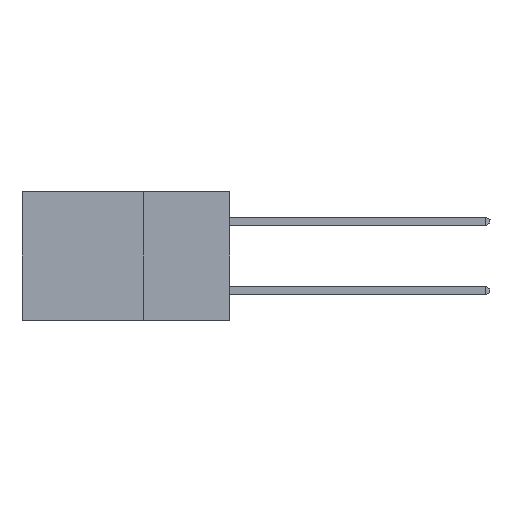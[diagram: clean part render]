
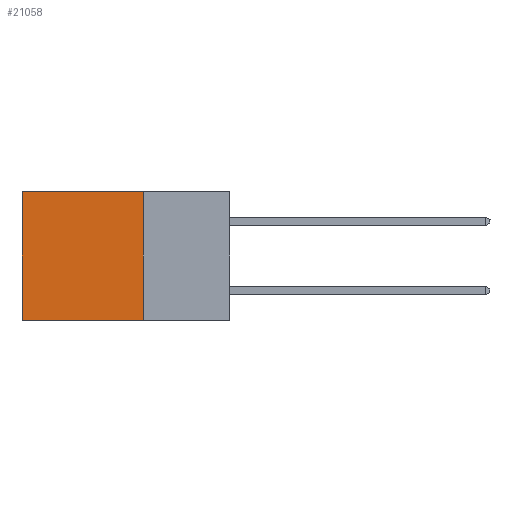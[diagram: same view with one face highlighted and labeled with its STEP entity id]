
A CAD part, left-side view. The second image highlights one B-rep face of the part: STEP entity #21058.
In plain terms, the highlighted planar face has unit normal (-1, 0, 0).
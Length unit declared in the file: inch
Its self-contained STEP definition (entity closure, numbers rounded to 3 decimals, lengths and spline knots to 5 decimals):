
#606 = DIRECTION ( 'NONE',  ( 0., 1., 0. ) ) ;
#782 = CARTESIAN_POINT ( 'NONE',  ( 0.298, 0.25, 0. ) ) ;
#2082 = VERTEX_POINT ( 'NONE', #9277 ) ;
#3116 = DIRECTION ( 'NONE',  ( 0., 0., -1. ) ) ;
#3853 = VECTOR ( 'NONE', #17124, 39.37008 ) ;
#4188 = ORIENTED_EDGE ( 'NONE', *, *, #10128, .F. ) ;
#5757 = VERTEX_POINT ( 'NONE', #782 ) ;
#6458 = CARTESIAN_POINT ( 'NONE',  ( 0.298, 0.6, 0. ) ) ;
#6996 = VERTEX_POINT ( 'NONE', #15014 ) ;
#7522 = LINE ( 'NONE', #8868, #10179 ) ;
#8371 = AXIS2_PLACEMENT_3D ( 'NONE', #20849, #12658, #12374 ) ;
#8868 = CARTESIAN_POINT ( 'NONE',  ( 0.298, 0.25, 0. ) ) ;
#9277 = CARTESIAN_POINT ( 'NONE',  ( 0.298, 0.6, -0.37 ) ) ;
#9330 = LINE ( 'NONE', #12622, #3853 ) ;
#9801 = DIRECTION ( 'NONE',  ( 0., 0., -1. ) ) ;
#9958 = ORIENTED_EDGE ( 'NONE', *, *, #11489, .T. ) ;
#10099 = CARTESIAN_POINT ( 'NONE',  ( 0.298, 0.25, 0. ) ) ;
#10128 = EDGE_CURVE ( 'NONE', #15564, #2082, #9330, .T. ) ;
#10179 = VECTOR ( 'NONE', #606, 39.37008 ) ;
#10204 = CARTESIAN_POINT ( 'NONE',  ( 0.298, 0.25, -0.37 ) ) ;
#10834 = LINE ( 'NONE', #6458, #21494 ) ;
#11045 = PLANE ( 'NONE',  #8371 ) ;
#11489 = EDGE_CURVE ( 'NONE', #6996, #2082, #10834, .T. ) ;
#12149 = LINE ( 'NONE', #10099, #16293 ) ;
#12374 = DIRECTION ( 'NONE',  ( 0., 0., -1. ) ) ;
#12622 = CARTESIAN_POINT ( 'NONE',  ( 0.298, 0.25, -0.37 ) ) ;
#12658 = DIRECTION ( 'NONE',  ( 1., 0., 0. ) ) ;
#13491 = FACE_OUTER_BOUND ( 'NONE', #16766, .T. ) ;
#14863 = EDGE_CURVE ( 'NONE', #5757, #15564, #12149, .T. ) ;
#15014 = CARTESIAN_POINT ( 'NONE',  ( 0.298, 0.6, 0. ) ) ;
#15564 = VERTEX_POINT ( 'NONE', #10204 ) ;
#16293 = VECTOR ( 'NONE', #9801, 39.37008 ) ;
#16766 = EDGE_LOOP ( 'NONE', ( #9958, #4188, #17423, #20135 ) ) ;
#17124 = DIRECTION ( 'NONE',  ( 0., 1., 0. ) ) ;
#17328 = EDGE_CURVE ( 'NONE', #5757, #6996, #7522, .T. ) ;
#17423 = ORIENTED_EDGE ( 'NONE', *, *, #14863, .F. ) ;
#20135 = ORIENTED_EDGE ( 'NONE', *, *, #17328, .T. ) ;
#20849 = CARTESIAN_POINT ( 'NONE',  ( 0.298, 0.25, 0. ) ) ;
#21058 = ADVANCED_FACE ( 'NONE', ( #13491 ), #11045, .F. ) ;
#21494 = VECTOR ( 'NONE', #3116, 39.37008 ) ;
